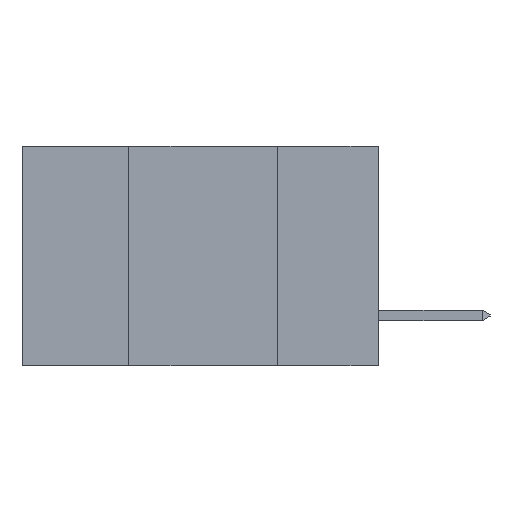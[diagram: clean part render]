
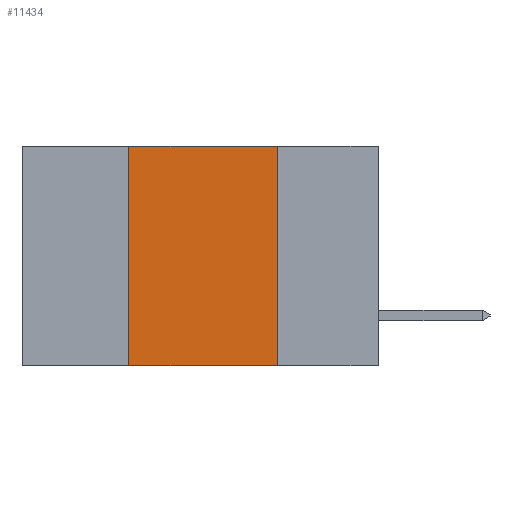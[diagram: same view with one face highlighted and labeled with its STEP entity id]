
A CAD part, left-side view. The second image highlights one B-rep face of the part: STEP entity #11434.
In plain terms, the highlighted planar face has unit normal (-1, 0, 0).
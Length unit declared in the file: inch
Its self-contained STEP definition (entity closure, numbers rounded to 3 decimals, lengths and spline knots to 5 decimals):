
#425 = EDGE_LOOP ( 'NONE', ( #3250, #1005, #5926, #10430 ) ) ;
#785 = LINE ( 'NONE', #1415, #7233 ) ;
#1005 = ORIENTED_EDGE ( 'NONE', *, *, #1468, .F. ) ;
#1138 = DIRECTION ( 'NONE',  ( 0., 0., -1. ) ) ;
#1356 = CARTESIAN_POINT ( 'NONE',  ( 0., 0.17, -0.37 ) ) ;
#1415 = CARTESIAN_POINT ( 'NONE',  ( 0., 0.6, 0. ) ) ;
#1458 = DIRECTION ( 'NONE',  ( 0., -1., 0. ) ) ;
#1468 = EDGE_CURVE ( 'NONE', #6756, #4485, #785, .T. ) ;
#1717 = DIRECTION ( 'NONE',  ( 0., 0., -1. ) ) ;
#2404 = FACE_OUTER_BOUND ( 'NONE', #425, .T. ) ;
#2936 = LINE ( 'NONE', #1356, #7133 ) ;
#2955 = VECTOR ( 'NONE', #9827, 39.37008 ) ;
#3250 = ORIENTED_EDGE ( 'NONE', *, *, #7649, .F. ) ;
#3378 = CARTESIAN_POINT ( 'NONE',  ( 0., 0.6, -0.37 ) ) ;
#4485 = VERTEX_POINT ( 'NONE', #10484 ) ;
#5525 = VERTEX_POINT ( 'NONE', #11321 ) ;
#5926 = ORIENTED_EDGE ( 'NONE', *, *, #6169, .F. ) ;
#6033 = CARTESIAN_POINT ( 'NONE',  ( 0., 0.17, -0.37 ) ) ;
#6086 = AXIS2_PLACEMENT_3D ( 'NONE', #8777, #7173, #1717 ) ;
#6169 = EDGE_CURVE ( 'NONE', #5525, #6756, #7682, .T. ) ;
#6289 = LINE ( 'NONE', #3378, #8542 ) ;
#6300 = PLANE ( 'NONE',  #6086 ) ;
#6756 = VERTEX_POINT ( 'NONE', #9286 ) ;
#7095 = DIRECTION ( 'NONE',  ( 0., -1., 0. ) ) ;
#7133 = VECTOR ( 'NONE', #1138, 39.37008 ) ;
#7173 = DIRECTION ( 'NONE',  ( 1., 0., 0. ) ) ;
#7233 = VECTOR ( 'NONE', #7095, 39.37008 ) ;
#7649 = EDGE_CURVE ( 'NONE', #4485, #10158, #2936, .T. ) ;
#7682 = LINE ( 'NONE', #9834, #2955 ) ;
#8542 = VECTOR ( 'NONE', #1458, 39.37008 ) ;
#8777 = CARTESIAN_POINT ( 'NONE',  ( 0., 0.6, 0. ) ) ;
#8957 = EDGE_CURVE ( 'NONE', #5525, #10158, #6289, .T. ) ;
#9286 = CARTESIAN_POINT ( 'NONE',  ( 0., 0.42, 0. ) ) ;
#9827 = DIRECTION ( 'NONE',  ( 0., 0., 1. ) ) ;
#9834 = CARTESIAN_POINT ( 'NONE',  ( 0., 0.42, -0.37 ) ) ;
#10158 = VERTEX_POINT ( 'NONE', #6033 ) ;
#10430 = ORIENTED_EDGE ( 'NONE', *, *, #8957, .T. ) ;
#10484 = CARTESIAN_POINT ( 'NONE',  ( 0., 0.17, 0. ) ) ;
#11321 = CARTESIAN_POINT ( 'NONE',  ( 0., 0.42, -0.37 ) ) ;
#11434 = ADVANCED_FACE ( 'NONE', ( #2404 ), #6300, .F. ) ;
